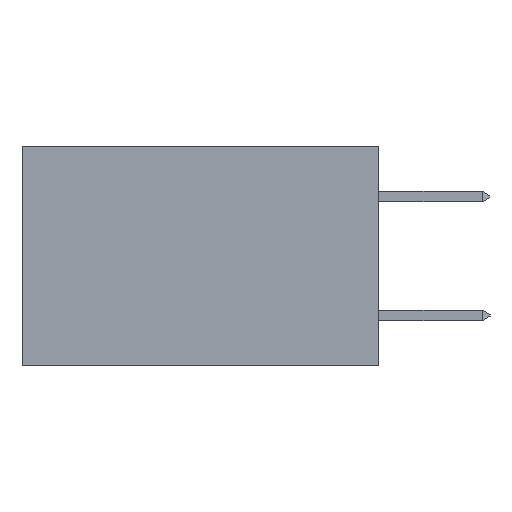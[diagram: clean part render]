
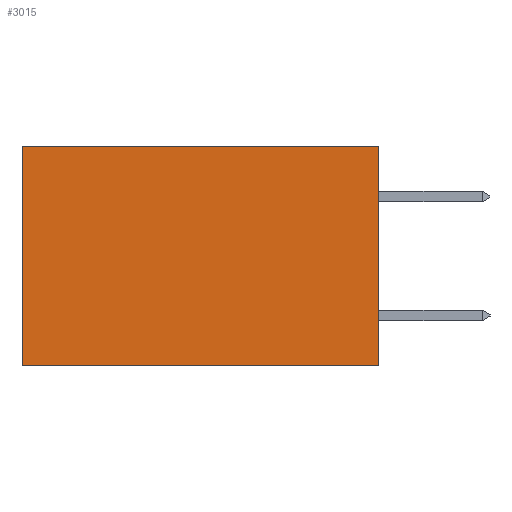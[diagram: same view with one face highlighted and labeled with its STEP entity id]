
A CAD part, left-side view. The second image highlights one B-rep face of the part: STEP entity #3015.
In plain terms, the highlighted planar face has unit normal (-1, 0, 0).
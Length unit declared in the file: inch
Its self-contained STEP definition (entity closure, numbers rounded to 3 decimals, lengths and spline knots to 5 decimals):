
#626 = CARTESIAN_POINT ( 'NONE',  ( 0.2615, 0., 0. ) ) ;
#641 = DIRECTION ( 'NONE',  ( 0., 1., 0. ) ) ;
#1102 = CARTESIAN_POINT ( 'NONE',  ( 0.2615, 0., 0. ) ) ;
#1138 = VECTOR ( 'NONE', #641, 39.37008 ) ;
#1403 = CARTESIAN_POINT ( 'NONE',  ( 0.2615, 0.6, -0.37 ) ) ;
#1766 = DIRECTION ( 'NONE',  ( 0., 0., -1. ) ) ;
#1871 = DIRECTION ( 'NONE',  ( 1., 0., 0. ) ) ;
#2405 = CARTESIAN_POINT ( 'NONE',  ( 0.2615, 0., -0.37 ) ) ;
#2683 = VERTEX_POINT ( 'NONE', #1102 ) ;
#3015 = ADVANCED_FACE ( 'NONE', ( #11480 ), #3776, .F. ) ;
#3096 = LINE ( 'NONE', #7865, #8986 ) ;
#3766 = CARTESIAN_POINT ( 'NONE',  ( 0.2615, 0., -0.37 ) ) ;
#3776 = PLANE ( 'NONE',  #13381 ) ;
#4493 = LINE ( 'NONE', #626, #1138 ) ;
#5713 = VERTEX_POINT ( 'NONE', #13552 ) ;
#6135 = VECTOR ( 'NONE', #9555, 39.37008 ) ;
#7337 = VERTEX_POINT ( 'NONE', #1403 ) ;
#7423 = EDGE_CURVE ( 'NONE', #2683, #5713, #4493, .T. ) ;
#7604 = EDGE_LOOP ( 'NONE', ( #8952, #9051, #9078, #13224 ) ) ;
#7779 = DIRECTION ( 'NONE',  ( 0., 1., 0. ) ) ;
#7865 = CARTESIAN_POINT ( 'NONE',  ( 0.2615, 0., -0.37 ) ) ;
#8158 = VECTOR ( 'NONE', #12932, 39.37008 ) ;
#8952 = ORIENTED_EDGE ( 'NONE', *, *, #12096, .T. ) ;
#8982 = EDGE_CURVE ( 'NONE', #13023, #7337, #3096, .T. ) ;
#8986 = VECTOR ( 'NONE', #7779, 39.37008 ) ;
#9051 = ORIENTED_EDGE ( 'NONE', *, *, #8982, .F. ) ;
#9078 = ORIENTED_EDGE ( 'NONE', *, *, #13708, .F. ) ;
#9555 = DIRECTION ( 'NONE',  ( 0., 0., -1. ) ) ;
#9581 = LINE ( 'NONE', #11395, #6135 ) ;
#11113 = LINE ( 'NONE', #11521, #8158 ) ;
#11395 = CARTESIAN_POINT ( 'NONE',  ( 0.2615, 0., -0.37 ) ) ;
#11480 = FACE_OUTER_BOUND ( 'NONE', #7604, .T. ) ;
#11521 = CARTESIAN_POINT ( 'NONE',  ( 0.2615, 0.6, -0.37 ) ) ;
#12096 = EDGE_CURVE ( 'NONE', #5713, #7337, #11113, .T. ) ;
#12932 = DIRECTION ( 'NONE',  ( 0., 0., -1. ) ) ;
#13023 = VERTEX_POINT ( 'NONE', #3766 ) ;
#13224 = ORIENTED_EDGE ( 'NONE', *, *, #7423, .T. ) ;
#13381 = AXIS2_PLACEMENT_3D ( 'NONE', #2405, #1871, #1766 ) ;
#13552 = CARTESIAN_POINT ( 'NONE',  ( 0.2615, 0.6, 0. ) ) ;
#13708 = EDGE_CURVE ( 'NONE', #2683, #13023, #9581, .T. ) ;
